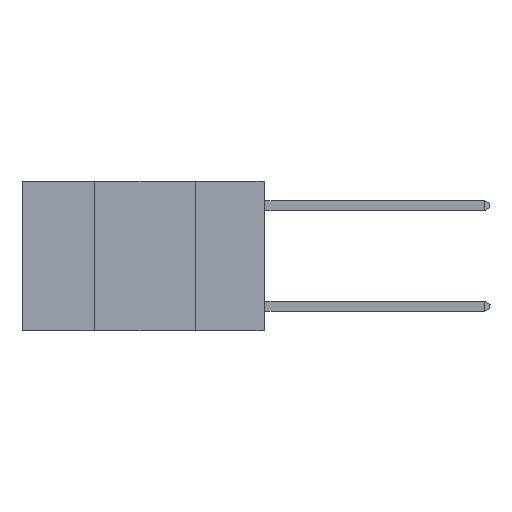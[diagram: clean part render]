
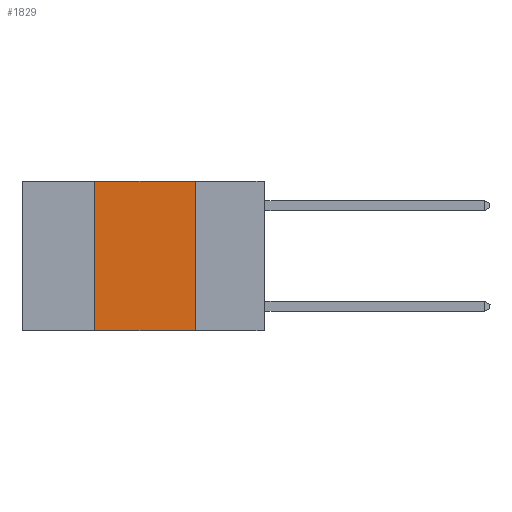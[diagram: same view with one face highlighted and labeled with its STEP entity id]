
A CAD part, left-side view. The second image highlights one B-rep face of the part: STEP entity #1829.
In plain terms, the highlighted planar face has unit normal (-1, 0, 0).
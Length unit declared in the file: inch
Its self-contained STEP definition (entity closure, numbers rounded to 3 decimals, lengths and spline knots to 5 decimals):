
#162 = VECTOR ( 'NONE', #6470, 39.37008 ) ;
#179 = CARTESIAN_POINT ( 'NONE',  ( 0., 0.42, 0. ) ) ;
#411 = LINE ( 'NONE', #5412, #11405 ) ;
#505 = LINE ( 'NONE', #1041, #162 ) ;
#1041 = CARTESIAN_POINT ( 'NONE',  ( 0., 0.17, 0. ) ) ;
#1336 = VERTEX_POINT ( 'NONE', #179 ) ;
#1360 = EDGE_LOOP ( 'NONE', ( #10152, #10897, #10592, #11614 ) ) ;
#1489 = DIRECTION ( 'NONE',  ( 1., 0., 0. ) ) ;
#1829 = ADVANCED_FACE ( 'NONE', ( #8311 ), #9953, .F. ) ;
#2515 = CARTESIAN_POINT ( 'NONE',  ( 0., 0.6, 0. ) ) ;
#2901 = CARTESIAN_POINT ( 'NONE',  ( 0., 0.42, -0.37 ) ) ;
#2968 = CARTESIAN_POINT ( 'NONE',  ( 0., 0.17, -0.37 ) ) ;
#3163 = CARTESIAN_POINT ( 'NONE',  ( 0., 0.6, 0. ) ) ;
#3377 = VERTEX_POINT ( 'NONE', #2901 ) ;
#4238 = EDGE_CURVE ( 'NONE', #3377, #8834, #411, .T. ) ;
#4888 = VERTEX_POINT ( 'NONE', #8642 ) ;
#5412 = CARTESIAN_POINT ( 'NONE',  ( 0., 0.6, -0.37 ) ) ;
#5416 = EDGE_CURVE ( 'NONE', #1336, #4888, #11033, .T. ) ;
#6470 = DIRECTION ( 'NONE',  ( 0., 0., -1. ) ) ;
#6771 = AXIS2_PLACEMENT_3D ( 'NONE', #2515, #1489, #9749 ) ;
#7528 = DIRECTION ( 'NONE',  ( 0., -1., 0. ) ) ;
#8033 = CARTESIAN_POINT ( 'NONE',  ( 0., 0.42, 0. ) ) ;
#8067 = VECTOR ( 'NONE', #7528, 39.37008 ) ;
#8311 = FACE_OUTER_BOUND ( 'NONE', #1360, .T. ) ;
#8616 = EDGE_CURVE ( 'NONE', #3377, #1336, #9596, .T. ) ;
#8642 = CARTESIAN_POINT ( 'NONE',  ( 0., 0.17, 0. ) ) ;
#8834 = VERTEX_POINT ( 'NONE', #2968 ) ;
#9596 = LINE ( 'NONE', #8033, #12248 ) ;
#9653 = EDGE_CURVE ( 'NONE', #4888, #8834, #505, .T. ) ;
#9749 = DIRECTION ( 'NONE',  ( 0., 0., -1. ) ) ;
#9846 = DIRECTION ( 'NONE',  ( 0., -1., 0. ) ) ;
#9953 = PLANE ( 'NONE',  #6771 ) ;
#10152 = ORIENTED_EDGE ( 'NONE', *, *, #9653, .F. ) ;
#10592 = ORIENTED_EDGE ( 'NONE', *, *, #8616, .F. ) ;
#10897 = ORIENTED_EDGE ( 'NONE', *, *, #5416, .F. ) ;
#11033 = LINE ( 'NONE', #3163, #8067 ) ;
#11405 = VECTOR ( 'NONE', #9846, 39.37008 ) ;
#11614 = ORIENTED_EDGE ( 'NONE', *, *, #4238, .T. ) ;
#12248 = VECTOR ( 'NONE', #13634, 39.37008 ) ;
#13634 = DIRECTION ( 'NONE',  ( 0., 0., 1. ) ) ;
